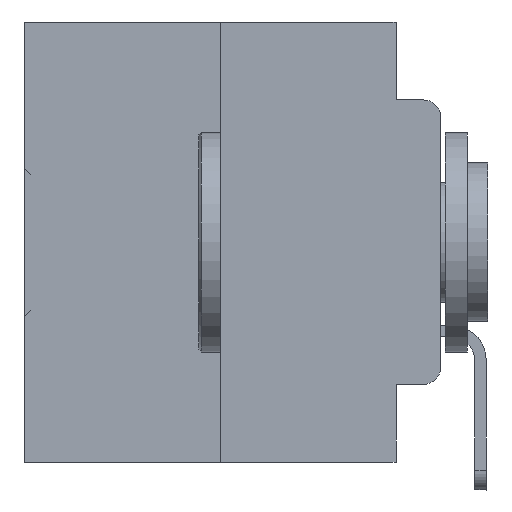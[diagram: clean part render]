
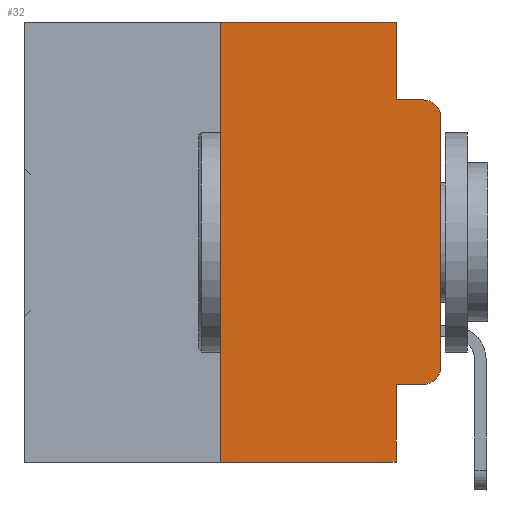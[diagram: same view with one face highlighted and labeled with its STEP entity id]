
A CAD part, left-side view. The second image highlights one B-rep face of the part: STEP entity #32.
In plain terms, the highlighted planar face has unit normal (-1, 0, 0).
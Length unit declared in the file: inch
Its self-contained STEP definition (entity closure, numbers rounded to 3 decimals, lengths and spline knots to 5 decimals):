
#32 = ADVANCED_FACE ( 'NONE', ( #16353 ), #2133, .F. ) ;
#43 = AXIS2_PLACEMENT_3D ( 'NONE', #18787, #27040, #2366 ) ;
#120 = VECTOR ( 'NONE', #33595, 39.37008 ) ;
#498 = DIRECTION ( 'NONE',  ( -1., 0., 0. ) ) ;
#621 = DIRECTION ( 'NONE',  ( 0., -1., 0. ) ) ;
#1079 = ORIENTED_EDGE ( 'NONE', *, *, #19923, .T. ) ;
#1181 = CARTESIAN_POINT ( 'NONE',  ( 0., 0.051, -0.0885 ) ) ;
#1810 = AXIS2_PLACEMENT_3D ( 'NONE', #11385, #498, #16919 ) ;
#2133 = PLANE ( 'NONE',  #43 ) ;
#2366 = DIRECTION ( 'NONE',  ( 0., 0., -1. ) ) ;
#2386 = LINE ( 'NONE', #21133, #30823 ) ;
#3542 = VECTOR ( 'NONE', #11254, 39.37008 ) ;
#3613 = DIRECTION ( 'NONE',  ( 0., 0., -1. ) ) ;
#3730 = CARTESIAN_POINT ( 'NONE',  ( 0., 0.473, 0. ) ) ;
#3843 = CARTESIAN_POINT ( 'NONE',  ( 0., 0.051, 0. ) ) ;
#4314 = LINE ( 'NONE', #15012, #22027 ) ;
#4653 = EDGE_CURVE ( 'NONE', #28425, #31421, #19719, .T. ) ;
#5359 = EDGE_CURVE ( 'NONE', #22576, #13892, #2386, .T. ) ;
#5723 = ORIENTED_EDGE ( 'NONE', *, *, #5359, .F. ) ;
#6072 = CIRCLE ( 'NONE', #1810, 0.02 ) ;
#6896 = CARTESIAN_POINT ( 'NONE',  ( 0., 0.473, -0.5 ) ) ;
#7098 = EDGE_CURVE ( 'NONE', #7944, #14231, #11775, .T. ) ;
#7574 = CARTESIAN_POINT ( 'NONE',  ( 0., 0.051, 0. ) ) ;
#7656 = EDGE_CURVE ( 'NONE', #27988, #7944, #20392, .T. ) ;
#7944 = VERTEX_POINT ( 'NONE', #1181 ) ;
#8624 = CARTESIAN_POINT ( 'NONE',  ( 0., 0., -0.3915 ) ) ;
#8675 = CARTESIAN_POINT ( 'NONE',  ( 0., 0.051, 0. ) ) ;
#8964 = EDGE_CURVE ( 'NONE', #23422, #23226, #28896, .T. ) ;
#9345 = ORIENTED_EDGE ( 'NONE', *, *, #4653, .T. ) ;
#9914 = EDGE_CURVE ( 'NONE', #22576, #23226, #31857, .T. ) ;
#10952 = LINE ( 'NONE', #28165, #120 ) ;
#11254 = DIRECTION ( 'NONE',  ( 0., -1., 0. ) ) ;
#11385 = CARTESIAN_POINT ( 'NONE',  ( 0., 0.02, -0.1085 ) ) ;
#11721 = VECTOR ( 'NONE', #3613, 39.37008 ) ;
#11775 = LINE ( 'NONE', #16423, #3542 ) ;
#12381 = CARTESIAN_POINT ( 'NONE',  ( 0., 0.02, -0.3915 ) ) ;
#13039 = VECTOR ( 'NONE', #25284, 39.37008 ) ;
#13564 = ORIENTED_EDGE ( 'NONE', *, *, #9914, .T. ) ;
#13892 = VERTEX_POINT ( 'NONE', #22936 ) ;
#14143 = ORIENTED_EDGE ( 'NONE', *, *, #35196, .F. ) ;
#14231 = VERTEX_POINT ( 'NONE', #33225 ) ;
#15012 = CARTESIAN_POINT ( 'NONE',  ( 0., 0.051, -0.4115 ) ) ;
#15400 = CARTESIAN_POINT ( 'NONE',  ( 0., 0., -0.1085 ) ) ;
#16353 = FACE_OUTER_BOUND ( 'NONE', #27074, .T. ) ;
#16423 = CARTESIAN_POINT ( 'NONE',  ( 0., 0.051, -0.0885 ) ) ;
#16913 = ORIENTED_EDGE ( 'NONE', *, *, #7656, .F. ) ;
#16919 = DIRECTION ( 'NONE',  ( 0., 0., -1. ) ) ;
#17048 = EDGE_CURVE ( 'NONE', #31421, #32772, #10952, .T. ) ;
#17693 = DIRECTION ( 'NONE',  ( -1., 0., 0. ) ) ;
#18787 = CARTESIAN_POINT ( 'NONE',  ( 0., 0.473, 0. ) ) ;
#19719 = CIRCLE ( 'NONE', #32495, 0.02 ) ;
#19923 = EDGE_CURVE ( 'NONE', #23422, #28425, #4314, .T. ) ;
#20392 = LINE ( 'NONE', #8675, #13039 ) ;
#20418 = EDGE_CURVE ( 'NONE', #32772, #14231, #6072, .T. ) ;
#20946 = DIRECTION ( 'NONE',  ( 0., 0., -1. ) ) ;
#21133 = CARTESIAN_POINT ( 'NONE',  ( 0., 0.25, 0. ) ) ;
#21410 = LINE ( 'NONE', #3730, #21817 ) ;
#21817 = VECTOR ( 'NONE', #621, 39.37008 ) ;
#22027 = VECTOR ( 'NONE', #25600, 39.37008 ) ;
#22576 = VERTEX_POINT ( 'NONE', #29215 ) ;
#22920 = ORIENTED_EDGE ( 'NONE', *, *, #20418, .T. ) ;
#22932 = CARTESIAN_POINT ( 'NONE',  ( 0., 0.051, -0.4115 ) ) ;
#22936 = CARTESIAN_POINT ( 'NONE',  ( 0., 0.25, 0. ) ) ;
#23226 = VERTEX_POINT ( 'NONE', #24145 ) ;
#23422 = VERTEX_POINT ( 'NONE', #22932 ) ;
#24145 = CARTESIAN_POINT ( 'NONE',  ( 0., 0.051, -0.5 ) ) ;
#24387 = CARTESIAN_POINT ( 'NONE',  ( 0., 0.02, -0.4115 ) ) ;
#24554 = VECTOR ( 'NONE', #28421, 39.37008 ) ;
#24802 = ORIENTED_EDGE ( 'NONE', *, *, #8964, .F. ) ;
#24975 = ORIENTED_EDGE ( 'NONE', *, *, #7098, .F. ) ;
#25284 = DIRECTION ( 'NONE',  ( 0., 0., -1. ) ) ;
#25600 = DIRECTION ( 'NONE',  ( 0., -1., 0. ) ) ;
#26846 = DIRECTION ( 'NONE',  ( 0., 0., 1. ) ) ;
#27040 = DIRECTION ( 'NONE',  ( 1., 0., 0. ) ) ;
#27074 = EDGE_LOOP ( 'NONE', ( #30782, #22920, #24975, #16913, #14143, #5723, #13564, #24802, #1079, #9345 ) ) ;
#27988 = VERTEX_POINT ( 'NONE', #7574 ) ;
#28165 = CARTESIAN_POINT ( 'NONE',  ( 0., 0., 0. ) ) ;
#28421 = DIRECTION ( 'NONE',  ( 0., -1., 0. ) ) ;
#28425 = VERTEX_POINT ( 'NONE', #24387 ) ;
#28896 = LINE ( 'NONE', #3843, #11721 ) ;
#29215 = CARTESIAN_POINT ( 'NONE',  ( 0., 0.25, -0.5 ) ) ;
#30782 = ORIENTED_EDGE ( 'NONE', *, *, #17048, .T. ) ;
#30823 = VECTOR ( 'NONE', #26846, 39.37008 ) ;
#31421 = VERTEX_POINT ( 'NONE', #8624 ) ;
#31857 = LINE ( 'NONE', #6896, #24554 ) ;
#32495 = AXIS2_PLACEMENT_3D ( 'NONE', #12381, #17693, #20946 ) ;
#32772 = VERTEX_POINT ( 'NONE', #15400 ) ;
#33225 = CARTESIAN_POINT ( 'NONE',  ( 0., 0.02, -0.0885 ) ) ;
#33595 = DIRECTION ( 'NONE',  ( 0., 0., 1. ) ) ;
#35196 = EDGE_CURVE ( 'NONE', #13892, #27988, #21410, .T. ) ;
